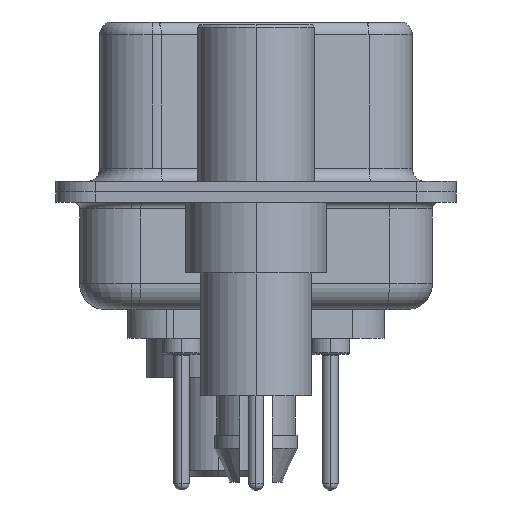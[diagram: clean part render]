
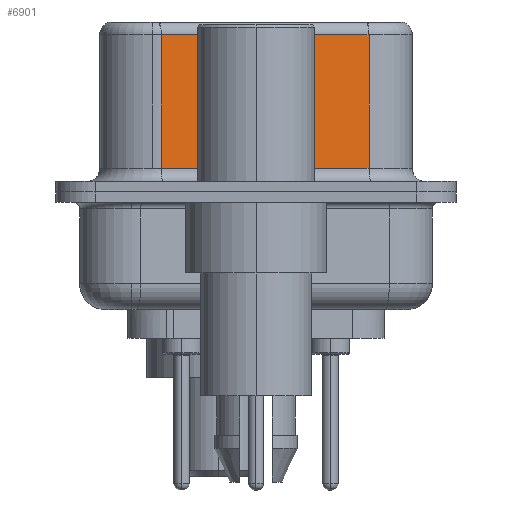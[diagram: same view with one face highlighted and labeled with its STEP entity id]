
A CAD part, left-side view. The second image highlights one B-rep face of the part: STEP entity #6901.
In plain terms, the highlighted planar face has unit normal (-0.985, -0.174, 0).
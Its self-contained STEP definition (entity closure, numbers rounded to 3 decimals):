
#1041 = DIRECTION ( 'NONE',  ( 0., 0., -1. ) ) ;
#1218 = EDGE_CURVE ( 'NONE', #16289, #25083, #27033, .T. ) ;
#1531 = CARTESIAN_POINT ( 'NONE',  ( 5.132, -4.322, 0.9 ) ) ;
#2099 = EDGE_CURVE ( 'NONE', #25083, #6119, #6838, .T. ) ;
#2499 = CARTESIAN_POINT ( 'NONE',  ( 5.132, -4.322, 6.52 ) ) ;
#2543 = VECTOR ( 'NONE', #11248, 1000. ) ;
#3447 = VECTOR ( 'NONE', #15135, 1000. ) ;
#4356 = EDGE_CURVE ( 'NONE', #6119, #12852, #9123, .T. ) ;
#4697 = CARTESIAN_POINT ( 'NONE',  ( 3.73, 3.628, 0.9 ) ) ;
#4735 = DIRECTION ( 'NONE',  ( 0., 0., -1. ) ) ;
#5609 = PLANE ( 'NONE',  #14147 ) ;
#6119 = VERTEX_POINT ( 'NONE', #4697 ) ;
#6803 = EDGE_LOOP ( 'NONE', ( #12777, #10509, #24658, #13639 ) ) ;
#6838 = LINE ( 'NONE', #25914, #17953 ) ;
#6901 = ADVANCED_FACE ( 'NONE', ( #21113 ), #5609, .F. ) ;
#7292 = EDGE_CURVE ( 'NONE', #16289, #12852, #13498, .T. ) ;
#7568 = VECTOR ( 'NONE', #4735, 1000. ) ;
#7836 = CARTESIAN_POINT ( 'NONE',  ( 5.132, -4.322, 6.52 ) ) ;
#8582 = CARTESIAN_POINT ( 'NONE',  ( 3.73, 3.628, 6.02 ) ) ;
#8917 = CARTESIAN_POINT ( 'NONE',  ( 5.132, -4.322, 6.02 ) ) ;
#9123 = LINE ( 'NONE', #11162, #2543 ) ;
#10068 = DIRECTION ( 'NONE',  ( -0.174, 0.985, 0. ) ) ;
#10509 = ORIENTED_EDGE ( 'NONE', *, *, #1218, .T. ) ;
#10811 = CARTESIAN_POINT ( 'NONE',  ( 5.132, -4.322, 6.02 ) ) ;
#11162 = CARTESIAN_POINT ( 'NONE',  ( 5.132, -4.322, 0.9 ) ) ;
#11248 = DIRECTION ( 'NONE',  ( 0.174, -0.985, 0. ) ) ;
#12777 = ORIENTED_EDGE ( 'NONE', *, *, #7292, .F. ) ;
#12852 = VERTEX_POINT ( 'NONE', #1531 ) ;
#13498 = LINE ( 'NONE', #2499, #7568 ) ;
#13639 = ORIENTED_EDGE ( 'NONE', *, *, #4356, .T. ) ;
#14147 = AXIS2_PLACEMENT_3D ( 'NONE', #7836, #23328, #10068 ) ;
#15135 = DIRECTION ( 'NONE',  ( -0.174, 0.985, 0. ) ) ;
#16289 = VERTEX_POINT ( 'NONE', #8917 ) ;
#17953 = VECTOR ( 'NONE', #1041, 1000. ) ;
#21113 = FACE_OUTER_BOUND ( 'NONE', #6803, .T. ) ;
#23328 = DIRECTION ( 'NONE',  ( 0.985, 0.174, 0. ) ) ;
#24658 = ORIENTED_EDGE ( 'NONE', *, *, #2099, .T. ) ;
#25083 = VERTEX_POINT ( 'NONE', #8582 ) ;
#25914 = CARTESIAN_POINT ( 'NONE',  ( 3.73, 3.628, 6.52 ) ) ;
#27033 = LINE ( 'NONE', #10811, #3447 ) ;
